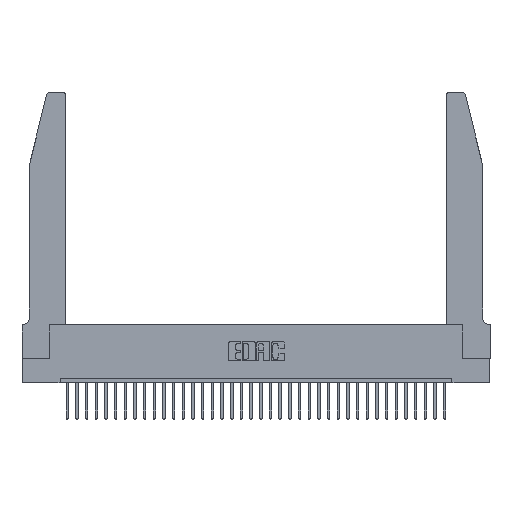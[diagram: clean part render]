
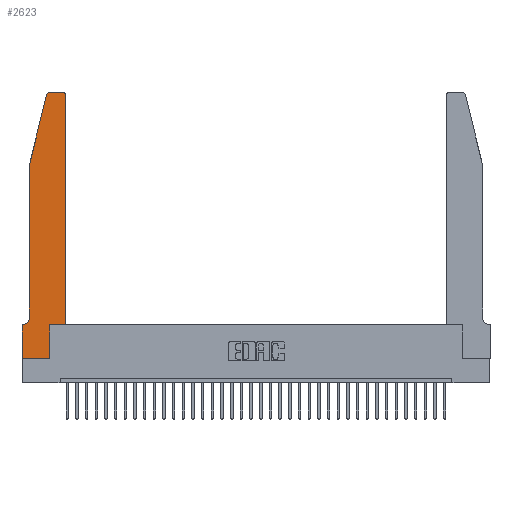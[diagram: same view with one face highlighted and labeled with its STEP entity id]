
A CAD part, top view. The second image highlights one B-rep face of the part: STEP entity #2623.
In plain terms, the highlighted planar face has unit normal (0, 0, 1).
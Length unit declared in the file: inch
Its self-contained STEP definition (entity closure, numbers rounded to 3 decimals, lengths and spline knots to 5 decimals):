
#68 = AXIS2_PLACEMENT_3D ( 'NONE', #4454, #22925, #25655 ) ;
#93 = DIRECTION ( 'NONE',  ( 0., 0., 1. ) ) ;
#1046 = DIRECTION ( 'NONE',  ( 1., 0., 0. ) ) ;
#1492 = DIRECTION ( 'NONE',  ( -0.239, -0.971, 0. ) ) ;
#2623 = ADVANCED_FACE ( 'NONE', ( #13248 ), #28708, .T. ) ;
#2672 = CARTESIAN_POINT ( 'NONE',  ( 0.284, 2.75, 0.37 ) ) ;
#3902 = LINE ( 'NONE', #12824, #17509 ) ;
#4197 = CARTESIAN_POINT ( 'NONE',  ( 0.4505, 2.72, 0.37 ) ) ;
#4365 = EDGE_CURVE ( 'NONE', #8148, #6129, #14967, .T. ) ;
#4454 = CARTESIAN_POINT ( 'NONE',  ( 0., 0.35, 0.37 ) ) ;
#5014 = DIRECTION ( 'NONE',  ( 0., -1., 0. ) ) ;
#5051 = EDGE_CURVE ( 'NONE', #31479, #26005, #13437, .T. ) ;
#5199 = VERTEX_POINT ( 'NONE', #7905 ) ;
#5369 = CARTESIAN_POINT ( 'NONE',  ( 0.0055, 0.42, 0.37 ) ) ;
#5797 = ORIENTED_EDGE ( 'NONE', *, *, #25515, .T. ) ;
#5977 = VECTOR ( 'NONE', #15652, 39.37008 ) ;
#6129 = VERTEX_POINT ( 'NONE', #19533 ) ;
#6265 = CARTESIAN_POINT ( 'NONE',  ( 0.0055, 0.35, 0.37 ) ) ;
#6359 = CARTESIAN_POINT ( 'NONE',  ( 0.2865, 0.35, 0.37 ) ) ;
#7415 = CARTESIAN_POINT ( 'NONE',  ( 0., 0., 0.37 ) ) ;
#7681 = EDGE_CURVE ( 'NONE', #32652, #19010, #9795, .T. ) ;
#7775 = ORIENTED_EDGE ( 'NONE', *, *, #4365, .T. ) ;
#7782 = CARTESIAN_POINT ( 'NONE',  ( 0.4205, 2.72, 0.37 ) ) ;
#7857 = VECTOR ( 'NONE', #10653, 39.37008 ) ;
#7905 = CARTESIAN_POINT ( 'NONE',  ( 0.4205, 2.75, 0.37 ) ) ;
#7907 = CARTESIAN_POINT ( 'NONE',  ( 0.2865, 0.35, 0.37 ) ) ;
#8148 = VERTEX_POINT ( 'NONE', #6359 ) ;
#8955 = EDGE_CURVE ( 'NONE', #33930, #12498, #28314, .T. ) ;
#9333 = VERTEX_POINT ( 'NONE', #2672 ) ;
#9795 = LINE ( 'NONE', #7415, #13598 ) ;
#10289 = ORIENTED_EDGE ( 'NONE', *, *, #13723, .T. ) ;
#10322 = DIRECTION ( 'NONE',  ( -1., 0., 0. ) ) ;
#10653 = DIRECTION ( 'NONE',  ( 0., 1., 0. ) ) ;
#10932 = EDGE_CURVE ( 'NONE', #19010, #14519, #26724, .T. ) ;
#11097 = CIRCLE ( 'NONE', #17979, 0.03 ) ;
#11304 = CARTESIAN_POINT ( 'NONE',  ( 0., 0., 0.37 ) ) ;
#11516 = LINE ( 'NONE', #21491, #5977 ) ;
#12498 = VERTEX_POINT ( 'NONE', #6265 ) ;
#12824 = CARTESIAN_POINT ( 'NONE',  ( 0.0755, 0.35, 0.37 ) ) ;
#13173 = ORIENTED_EDGE ( 'NONE', *, *, #27638, .T. ) ;
#13248 = FACE_OUTER_BOUND ( 'NONE', #31754, .T. ) ;
#13437 = LINE ( 'NONE', #18001, #34543 ) ;
#13598 = VECTOR ( 'NONE', #5014, 39.37008 ) ;
#13708 = DIRECTION ( 'NONE',  ( 1., 0., 0. ) ) ;
#13723 = EDGE_CURVE ( 'NONE', #14519, #8148, #16755, .T. ) ;
#13724 = CARTESIAN_POINT ( 'NONE',  ( 0.0755, 2., 0.37 ) ) ;
#14121 = ORIENTED_EDGE ( 'NONE', *, *, #5051, .T. ) ;
#14519 = VERTEX_POINT ( 'NONE', #14560 ) ;
#14560 = CARTESIAN_POINT ( 'NONE',  ( 0.2865, 0., 0.37 ) ) ;
#14967 = LINE ( 'NONE', #17328, #34821 ) ;
#15652 = DIRECTION ( 'NONE',  ( 0., -1., 0. ) ) ;
#15983 = LINE ( 'NONE', #34437, #34963 ) ;
#16208 = DIRECTION ( 'NONE',  ( 0., 1., 0. ) ) ;
#16227 = ORIENTED_EDGE ( 'NONE', *, *, #17629, .T. ) ;
#16233 = CIRCLE ( 'NONE', #31251, 0.03 ) ;
#16755 = LINE ( 'NONE', #7907, #7857 ) ;
#16773 = LINE ( 'NONE', #32387, #33691 ) ;
#17328 = CARTESIAN_POINT ( 'NONE',  ( 0.4505, 0.35, 0.37 ) ) ;
#17509 = VECTOR ( 'NONE', #26393, 39.37008 ) ;
#17629 = EDGE_CURVE ( 'NONE', #9333, #31479, #11097, .T. ) ;
#17979 = AXIS2_PLACEMENT_3D ( 'NONE', #23286, #26011, #28104 ) ;
#18001 = CARTESIAN_POINT ( 'NONE',  ( 0.0755, 2., 0.37 ) ) ;
#18428 = CARTESIAN_POINT ( 'NONE',  ( 0.25487, 2.72718, 0.37 ) ) ;
#18685 = VECTOR ( 'NONE', #32895, 39.37008 ) ;
#18899 = ORIENTED_EDGE ( 'NONE', *, *, #33437, .T. ) ;
#19010 = VERTEX_POINT ( 'NONE', #11304 ) ;
#19533 = CARTESIAN_POINT ( 'NONE',  ( 0.4505, 0.35, 0.37 ) ) ;
#20161 = ORIENTED_EDGE ( 'NONE', *, *, #20911, .T. ) ;
#20911 = EDGE_CURVE ( 'NONE', #6129, #33292, #16773, .T. ) ;
#21491 = CARTESIAN_POINT ( 'NONE',  ( 0.0755, 2., 0.37 ) ) ;
#22145 = ORIENTED_EDGE ( 'NONE', *, *, #7681, .T. ) ;
#22925 = DIRECTION ( 'NONE',  ( 0., 0., 1. ) ) ;
#23286 = CARTESIAN_POINT ( 'NONE',  ( 0.284, 2.72, 0.37 ) ) ;
#25515 = EDGE_CURVE ( 'NONE', #5199, #9333, #15983, .T. ) ;
#25655 = DIRECTION ( 'NONE',  ( 1., 0., 0. ) ) ;
#25696 = CARTESIAN_POINT ( 'NONE',  ( 0.0755, 0.42, 0.37 ) ) ;
#26005 = VERTEX_POINT ( 'NONE', #13724 ) ;
#26011 = DIRECTION ( 'NONE',  ( 0., 0., 1. ) ) ;
#26393 = DIRECTION ( 'NONE',  ( -1., 0., 0. ) ) ;
#26724 = LINE ( 'NONE', #30052, #18685 ) ;
#26792 = ORIENTED_EDGE ( 'NONE', *, *, #10932, .T. ) ;
#27212 = EDGE_CURVE ( 'NONE', #12498, #32652, #3902, .T. ) ;
#27638 = EDGE_CURVE ( 'NONE', #33292, #5199, #16233, .T. ) ;
#28104 = DIRECTION ( 'NONE',  ( 1., 0., 0. ) ) ;
#28314 = CIRCLE ( 'NONE', #30910, 0.07 ) ;
#28708 = PLANE ( 'NONE',  #68 ) ;
#29495 = DIRECTION ( 'NONE',  ( -1., 0., 0. ) ) ;
#29851 = ORIENTED_EDGE ( 'NONE', *, *, #8955, .T. ) ;
#30052 = CARTESIAN_POINT ( 'NONE',  ( 0., 0., 0.37 ) ) ;
#30910 = AXIS2_PLACEMENT_3D ( 'NONE', #5369, #35072, #29495 ) ;
#31097 = ORIENTED_EDGE ( 'NONE', *, *, #27212, .T. ) ;
#31251 = AXIS2_PLACEMENT_3D ( 'NONE', #7782, #93, #13708 ) ;
#31479 = VERTEX_POINT ( 'NONE', #18428 ) ;
#31754 = EDGE_LOOP ( 'NONE', ( #5797, #16227, #14121, #18899, #29851, #31097, #22145, #26792, #10289, #7775, #20161, #13173 ) ) ;
#32387 = CARTESIAN_POINT ( 'NONE',  ( 0.4505, 0.35, 0.37 ) ) ;
#32652 = VERTEX_POINT ( 'NONE', #34439 ) ;
#32895 = DIRECTION ( 'NONE',  ( 1., 0., 0. ) ) ;
#33292 = VERTEX_POINT ( 'NONE', #4197 ) ;
#33437 = EDGE_CURVE ( 'NONE', #26005, #33930, #11516, .T. ) ;
#33691 = VECTOR ( 'NONE', #16208, 39.37008 ) ;
#33930 = VERTEX_POINT ( 'NONE', #25696 ) ;
#34437 = CARTESIAN_POINT ( 'NONE',  ( 0.2605, 2.75, 0.37 ) ) ;
#34439 = CARTESIAN_POINT ( 'NONE',  ( 0., 0.35, 0.37 ) ) ;
#34543 = VECTOR ( 'NONE', #1492, 39.37008 ) ;
#34821 = VECTOR ( 'NONE', #1046, 39.37008 ) ;
#34963 = VECTOR ( 'NONE', #10322, 39.37008 ) ;
#35072 = DIRECTION ( 'NONE',  ( 0., 0., -1. ) ) ;
